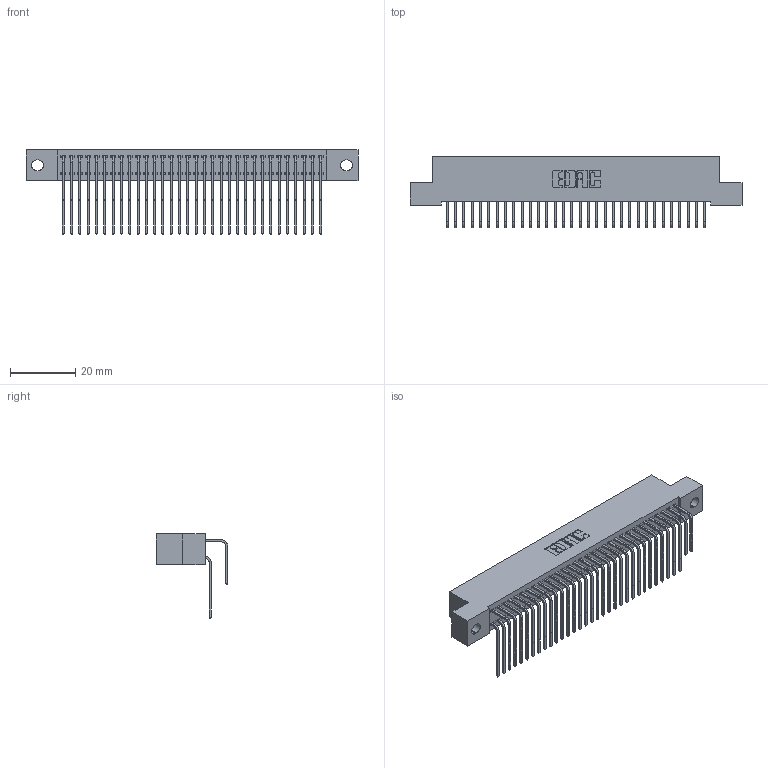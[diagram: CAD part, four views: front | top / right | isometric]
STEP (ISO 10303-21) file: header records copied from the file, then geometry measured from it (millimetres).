
FILE_DESCRIPTION (( 'STEP AP203' ), '1' );
FILE_NAME ('392-064-558-202.STEP', '2018-08-17T21:53:17', ( '' ), ( '' ), 'SwSTEP 2.0', 'SolidWorks 2016', '' );
FILE_SCHEMA (( 'CONFIG_CONTROL_DESIGN' ));
Length unit declared in the file: inch
Products named in the file (4): 342 Part_.128 Slot; 345-292-001_558 559 Tail - 1; 345-292-001_558 Tail - 2; 392-064-558-202
Assembly tree (65 placements, depth 2):
  392-064-558-202
    342 Part_.128 Slot
    345-292-001_558 559 Tail - 1  x32
    345-292-001_558 Tail - 2  x32
Bounding box: 101.6 x 21.91 x 25.78 mm (x, y, z)
Volume: 9398.5 mm3; surface area: 16481.6 mm2
Topology: 65 solids, 65 shells, 3570 faces, 10615 edges, 6990 vertices
Faces by surface type: plane 2502, cylinder 1068
Entity records: 23667 total; most frequent: CARTESIAN_POINT 3985, ORIENTED_EDGE 3870, DIRECTION 3403, EDGE_CURVE 1935, VECTOR 1767, LINE 1767, VERTEX_POINT 1286, AXIS2_PLACEMENT_3D 818
